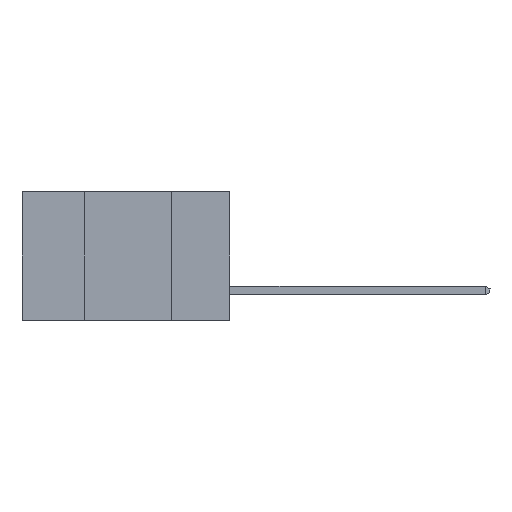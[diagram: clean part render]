
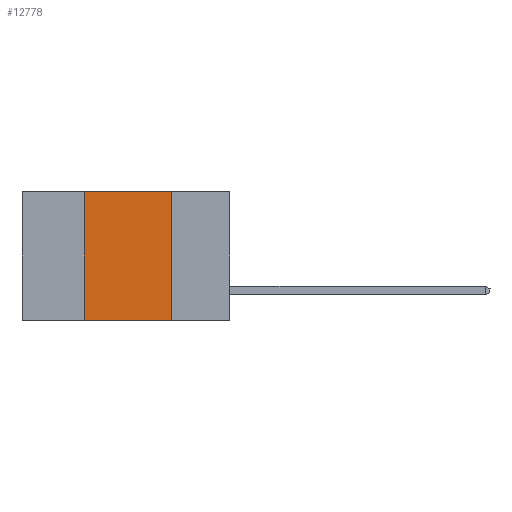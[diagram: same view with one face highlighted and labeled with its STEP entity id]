
A CAD part, left-side view. The second image highlights one B-rep face of the part: STEP entity #12778.
In plain terms, the highlighted planar face has unit normal (-1, 0, 0).
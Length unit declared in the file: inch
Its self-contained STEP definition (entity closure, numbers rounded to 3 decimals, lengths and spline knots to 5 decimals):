
#423 = CARTESIAN_POINT ( 'NONE',  ( 0., 0.6, -0.37 ) ) ;
#545 = CARTESIAN_POINT ( 'NONE',  ( 0., 0.17, 0. ) ) ;
#1235 = VERTEX_POINT ( 'NONE', #545 ) ;
#1520 = CARTESIAN_POINT ( 'NONE',  ( 0., 0.6, 0. ) ) ;
#2151 = CARTESIAN_POINT ( 'NONE',  ( 0., 0.17, -0.37 ) ) ;
#2469 = DIRECTION ( 'NONE',  ( 0., -1., 0. ) ) ;
#3363 = CARTESIAN_POINT ( 'NONE',  ( 0., 0.6, 0. ) ) ;
#3462 = PLANE ( 'NONE',  #16507 ) ;
#3468 = DIRECTION ( 'NONE',  ( 0., -1., 0. ) ) ;
#3517 = VERTEX_POINT ( 'NONE', #16242 ) ;
#3973 = ORIENTED_EDGE ( 'NONE', *, *, #13788, .T. ) ;
#4254 = ORIENTED_EDGE ( 'NONE', *, *, #17327, .F. ) ;
#5452 = VERTEX_POINT ( 'NONE', #18782 ) ;
#5685 = EDGE_LOOP ( 'NONE', ( #8955, #4254, #18994, #3973 ) ) ;
#7968 = CARTESIAN_POINT ( 'NONE',  ( 0., 0.42, -0.37 ) ) ;
#8955 = ORIENTED_EDGE ( 'NONE', *, *, #10175, .F. ) ;
#9335 = LINE ( 'NONE', #7968, #18843 ) ;
#9447 = FACE_OUTER_BOUND ( 'NONE', #5685, .T. ) ;
#9559 = VECTOR ( 'NONE', #11627, 39.37008 ) ;
#9753 = DIRECTION ( 'NONE',  ( 0., 0., -1. ) ) ;
#10175 = EDGE_CURVE ( 'NONE', #1235, #13828, #14793, .T. ) ;
#11627 = DIRECTION ( 'NONE',  ( 0., 0., -1. ) ) ;
#11929 = CARTESIAN_POINT ( 'NONE',  ( 0., 0.17, -0.37 ) ) ;
#12447 = DIRECTION ( 'NONE',  ( 1., 0., 0. ) ) ;
#12778 = ADVANCED_FACE ( 'NONE', ( #9447 ), #3462, .F. ) ;
#13788 = EDGE_CURVE ( 'NONE', #3517, #13828, #18125, .T. ) ;
#13828 = VERTEX_POINT ( 'NONE', #11929 ) ;
#14793 = LINE ( 'NONE', #2151, #9559 ) ;
#16242 = CARTESIAN_POINT ( 'NONE',  ( 0., 0.42, -0.37 ) ) ;
#16507 = AXIS2_PLACEMENT_3D ( 'NONE', #1520, #12447, #9753 ) ;
#16866 = VECTOR ( 'NONE', #2469, 39.37008 ) ;
#17195 = VECTOR ( 'NONE', #3468, 39.37008 ) ;
#17327 = EDGE_CURVE ( 'NONE', #5452, #1235, #19036, .T. ) ;
#18125 = LINE ( 'NONE', #423, #16866 ) ;
#18632 = DIRECTION ( 'NONE',  ( 0., 0., 1. ) ) ;
#18782 = CARTESIAN_POINT ( 'NONE',  ( 0., 0.42, 0. ) ) ;
#18843 = VECTOR ( 'NONE', #18632, 39.37008 ) ;
#18844 = EDGE_CURVE ( 'NONE', #3517, #5452, #9335, .T. ) ;
#18994 = ORIENTED_EDGE ( 'NONE', *, *, #18844, .F. ) ;
#19036 = LINE ( 'NONE', #3363, #17195 ) ;
